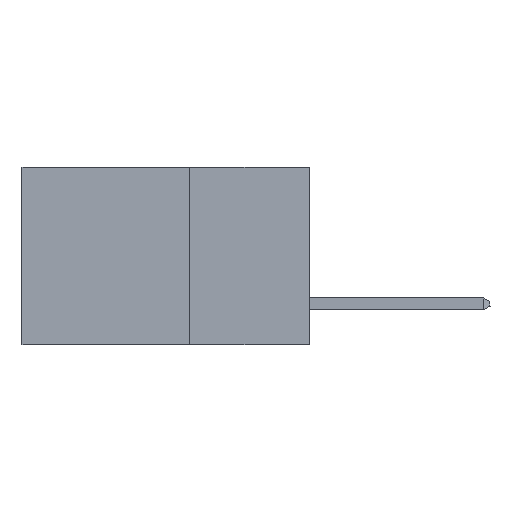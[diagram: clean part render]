
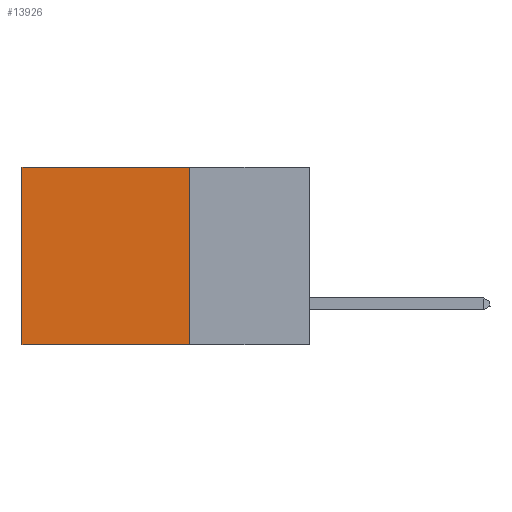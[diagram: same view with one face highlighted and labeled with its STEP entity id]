
A CAD part, left-side view. The second image highlights one B-rep face of the part: STEP entity #13926.
In plain terms, the highlighted planar face has unit normal (-1, 0, 0).
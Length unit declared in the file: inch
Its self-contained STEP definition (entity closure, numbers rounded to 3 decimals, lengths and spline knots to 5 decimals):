
#760 = ORIENTED_EDGE ( 'NONE', *, *, #17271, .F. ) ;
#1561 = FACE_OUTER_BOUND ( 'NONE', #14952, .T. ) ;
#1741 = EDGE_CURVE ( 'NONE', #4134, #4836, #17606, .T. ) ;
#2747 = DIRECTION ( 'NONE',  ( 1., 0., 0. ) ) ;
#4134 = VERTEX_POINT ( 'NONE', #11559 ) ;
#4489 = VECTOR ( 'NONE', #23978, 39.37008 ) ;
#4570 = ORIENTED_EDGE ( 'NONE', *, *, #8802, .T. ) ;
#4836 = VERTEX_POINT ( 'NONE', #24573 ) ;
#5036 = ORIENTED_EDGE ( 'NONE', *, *, #1741, .F. ) ;
#5791 = EDGE_CURVE ( 'NONE', #18967, #28322, #23877, .T. ) ;
#6676 = CARTESIAN_POINT ( 'NONE',  ( 0.2875, 0.6, 0. ) ) ;
#6969 = DIRECTION ( 'NONE',  ( 0., 0., -1. ) ) ;
#8562 = CARTESIAN_POINT ( 'NONE',  ( 0.2875, 0.25, 0. ) ) ;
#8802 = EDGE_CURVE ( 'NONE', #4134, #18967, #28075, .T. ) ;
#9957 = DIRECTION ( 'NONE',  ( 0., 1., 0. ) ) ;
#10669 = CARTESIAN_POINT ( 'NONE',  ( 0.2875, 0.25, 0. ) ) ;
#11435 = VECTOR ( 'NONE', #17314, 39.37008 ) ;
#11559 = CARTESIAN_POINT ( 'NONE',  ( 0.2875, 0.25, 0. ) ) ;
#12850 = VECTOR ( 'NONE', #22136, 39.37008 ) ;
#13926 = ADVANCED_FACE ( 'NONE', ( #1561 ), #20495, .F. ) ;
#14356 = AXIS2_PLACEMENT_3D ( 'NONE', #22602, #2747, #6969 ) ;
#14952 = EDGE_LOOP ( 'NONE', ( #26824, #760, #5036, #4570 ) ) ;
#15721 = CARTESIAN_POINT ( 'NONE',  ( 0.2875, 0.6, -0.37 ) ) ;
#17271 = EDGE_CURVE ( 'NONE', #4836, #28322, #27860, .T. ) ;
#17314 = DIRECTION ( 'NONE',  ( 0., 1., 0. ) ) ;
#17606 = LINE ( 'NONE', #8562, #4489 ) ;
#18522 = VECTOR ( 'NONE', #9957, 39.37008 ) ;
#18561 = CARTESIAN_POINT ( 'NONE',  ( 0.2875, 0.25, -0.37 ) ) ;
#18967 = VERTEX_POINT ( 'NONE', #28459 ) ;
#20495 = PLANE ( 'NONE',  #14356 ) ;
#22136 = DIRECTION ( 'NONE',  ( 0., 0., -1. ) ) ;
#22602 = CARTESIAN_POINT ( 'NONE',  ( 0.2875, 0.25, 0. ) ) ;
#23877 = LINE ( 'NONE', #6676, #12850 ) ;
#23978 = DIRECTION ( 'NONE',  ( 0., 0., -1. ) ) ;
#24573 = CARTESIAN_POINT ( 'NONE',  ( 0.2875, 0.25, -0.37 ) ) ;
#26824 = ORIENTED_EDGE ( 'NONE', *, *, #5791, .T. ) ;
#27860 = LINE ( 'NONE', #18561, #18522 ) ;
#28075 = LINE ( 'NONE', #10669, #11435 ) ;
#28322 = VERTEX_POINT ( 'NONE', #15721 ) ;
#28459 = CARTESIAN_POINT ( 'NONE',  ( 0.2875, 0.6, 0. ) ) ;
